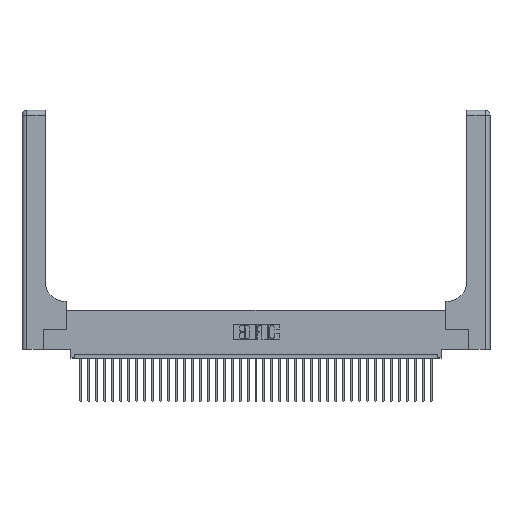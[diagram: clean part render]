
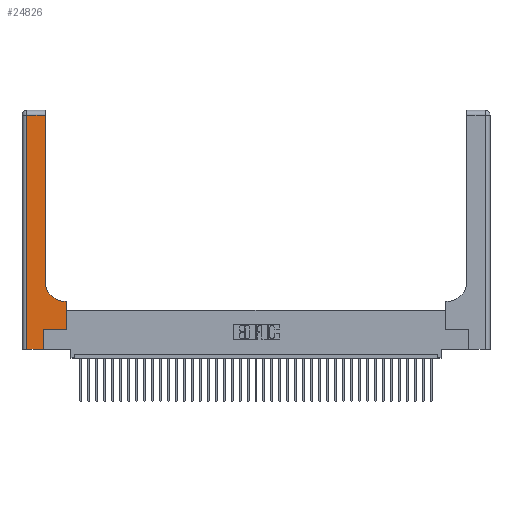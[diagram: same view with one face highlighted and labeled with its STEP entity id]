
A CAD part, top view. The second image highlights one B-rep face of the part: STEP entity #24826.
In plain terms, the highlighted planar face has unit normal (0, 0, 1).
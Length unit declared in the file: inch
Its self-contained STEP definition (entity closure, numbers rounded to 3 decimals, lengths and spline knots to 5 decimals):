
#1493 = VERTEX_POINT ( 'NONE', #10983 ) ;
#1577 = CARTESIAN_POINT ( 'NONE',  ( 0.269, 0., 0.37 ) ) ;
#2218 = CARTESIAN_POINT ( 'NONE',  ( 0., 0., 0.37 ) ) ;
#2765 = EDGE_LOOP ( 'NONE', ( #13888, #10366, #20046, #31240, #20888, #6402, #36610, #22506, #7918 ) ) ;
#3452 = DIRECTION ( 'NONE',  ( -1., 0., 0. ) ) ;
#3669 = EDGE_CURVE ( 'NONE', #20541, #1493, #30963, .T. ) ;
#4000 = EDGE_CURVE ( 'NONE', #6047, #23881, #18734, .T. ) ;
#4711 = VERTEX_POINT ( 'NONE', #16500 ) ;
#5059 = FACE_OUTER_BOUND ( 'NONE', #2765, .T. ) ;
#6047 = VERTEX_POINT ( 'NONE', #29308 ) ;
#6402 = ORIENTED_EDGE ( 'NONE', *, *, #3669, .T. ) ;
#6941 = CARTESIAN_POINT ( 'NONE',  ( 0., 3., 0.37 ) ) ;
#7346 = EDGE_CURVE ( 'NONE', #23881, #21358, #34104, .T. ) ;
#7569 = DIRECTION ( 'NONE',  ( 0., 1., 0. ) ) ;
#7597 = VERTEX_POINT ( 'NONE', #26483 ) ;
#7918 = ORIENTED_EDGE ( 'NONE', *, *, #4000, .T. ) ;
#8525 = CARTESIAN_POINT ( 'NONE',  ( 0.2915, 0.85, 0.37 ) ) ;
#8755 = VECTOR ( 'NONE', #35347, 39.37008 ) ;
#10366 = ORIENTED_EDGE ( 'NONE', *, *, #23251, .T. ) ;
#10983 = CARTESIAN_POINT ( 'NONE',  ( 0.5585, 0.25, 0.37 ) ) ;
#11232 = CARTESIAN_POINT ( 'NONE',  ( 0.2915, 2.94, 0.37 ) ) ;
#11728 = CARTESIAN_POINT ( 'NONE',  ( 0.06, 2.94, 0.37 ) ) ;
#12979 = LINE ( 'NONE', #2218, #8755 ) ;
#13381 = EDGE_CURVE ( 'NONE', #4711, #6047, #32341, .T. ) ;
#13420 = VERTEX_POINT ( 'NONE', #27987 ) ;
#13888 = ORIENTED_EDGE ( 'NONE', *, *, #7346, .T. ) ;
#13930 = CARTESIAN_POINT ( 'NONE',  ( 0.269, 0.25, 0.37 ) ) ;
#14029 = VECTOR ( 'NONE', #29819, 39.37008 ) ;
#14521 = DIRECTION ( 'NONE',  ( 0., 0., -1. ) ) ;
#14661 = CARTESIAN_POINT ( 'NONE',  ( 0.5415, 0.85, 0.37 ) ) ;
#16177 = EDGE_CURVE ( 'NONE', #13420, #20541, #23651, .T. ) ;
#16437 = LINE ( 'NONE', #27366, #28647 ) ;
#16500 = CARTESIAN_POINT ( 'NONE',  ( 0.5585, 0.6, 0.37 ) ) ;
#17772 = VECTOR ( 'NONE', #33254, 39.37008 ) ;
#17928 = DIRECTION ( 'NONE',  ( 0., -1., 0. ) ) ;
#18734 = CIRCLE ( 'NONE', #19576, 0.25 ) ;
#19576 = AXIS2_PLACEMENT_3D ( 'NONE', #14661, #14521, #35503 ) ;
#19998 = CARTESIAN_POINT ( 'NONE',  ( 0.2915, 0.6, 0.37 ) ) ;
#20046 = ORIENTED_EDGE ( 'NONE', *, *, #22298, .T. ) ;
#20131 = DIRECTION ( 'NONE',  ( -1., 0., 0. ) ) ;
#20541 = VERTEX_POINT ( 'NONE', #23118 ) ;
#20730 = DIRECTION ( 'NONE',  ( 0., 1., 0. ) ) ;
#20888 = ORIENTED_EDGE ( 'NONE', *, *, #16177, .T. ) ;
#21358 = VERTEX_POINT ( 'NONE', #11232 ) ;
#22298 = EDGE_CURVE ( 'NONE', #28649, #7597, #36614, .T. ) ;
#22325 = EDGE_CURVE ( 'NONE', #1493, #4711, #16437, .T. ) ;
#22506 = ORIENTED_EDGE ( 'NONE', *, *, #13381, .T. ) ;
#22922 = LINE ( 'NONE', #32995, #17772 ) ;
#22964 = VECTOR ( 'NONE', #20131, 39.37008 ) ;
#23118 = CARTESIAN_POINT ( 'NONE',  ( 0.269, 0.25, 0.37 ) ) ;
#23251 = EDGE_CURVE ( 'NONE', #21358, #28649, #22922, .T. ) ;
#23651 = LINE ( 'NONE', #1577, #31632 ) ;
#23881 = VERTEX_POINT ( 'NONE', #8525 ) ;
#24826 = ADVANCED_FACE ( 'NONE', ( #5059 ), #27912, .F. ) ;
#24889 = VECTOR ( 'NONE', #17928, 39.37008 ) ;
#25216 = EDGE_CURVE ( 'NONE', #7597, #13420, #12979, .T. ) ;
#25217 = VECTOR ( 'NONE', #20730, 39.37008 ) ;
#26483 = CARTESIAN_POINT ( 'NONE',  ( 0.06, 0., 0.37 ) ) ;
#27366 = CARTESIAN_POINT ( 'NONE',  ( 0.5585, 0.25, 0.37 ) ) ;
#27912 = PLANE ( 'NONE',  #35440 ) ;
#27987 = CARTESIAN_POINT ( 'NONE',  ( 0.269, 0., 0.37 ) ) ;
#28647 = VECTOR ( 'NONE', #30380, 39.37008 ) ;
#28649 = VERTEX_POINT ( 'NONE', #11728 ) ;
#29308 = CARTESIAN_POINT ( 'NONE',  ( 0.5415, 0.6, 0.37 ) ) ;
#29819 = DIRECTION ( 'NONE',  ( 1., 0., 0. ) ) ;
#30380 = DIRECTION ( 'NONE',  ( 0., 1., 0. ) ) ;
#30430 = DIRECTION ( 'NONE',  ( 0., 0., -1. ) ) ;
#30963 = LINE ( 'NONE', #13930, #14029 ) ;
#31240 = ORIENTED_EDGE ( 'NONE', *, *, #25216, .T. ) ;
#31632 = VECTOR ( 'NONE', #7569, 39.37008 ) ;
#32341 = LINE ( 'NONE', #19998, #22964 ) ;
#32995 = CARTESIAN_POINT ( 'NONE',  ( 0., 2.94, 0.37 ) ) ;
#33254 = DIRECTION ( 'NONE',  ( -1., 0., 0. ) ) ;
#34104 = LINE ( 'NONE', #38634, #25217 ) ;
#35347 = DIRECTION ( 'NONE',  ( 1., 0., 0. ) ) ;
#35440 = AXIS2_PLACEMENT_3D ( 'NONE', #6941, #30430, #3452 ) ;
#35503 = DIRECTION ( 'NONE',  ( 1., 0., 0. ) ) ;
#36270 = CARTESIAN_POINT ( 'NONE',  ( 0.06, 3., 0.37 ) ) ;
#36610 = ORIENTED_EDGE ( 'NONE', *, *, #22325, .T. ) ;
#36614 = LINE ( 'NONE', #36270, #24889 ) ;
#38634 = CARTESIAN_POINT ( 'NONE',  ( 0.2915, 3., 0.37 ) ) ;
